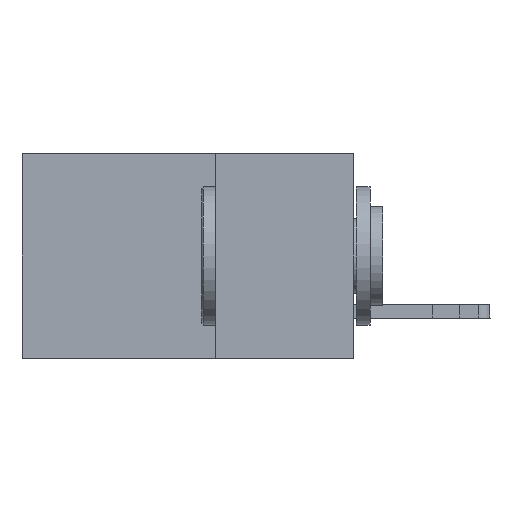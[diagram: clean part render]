
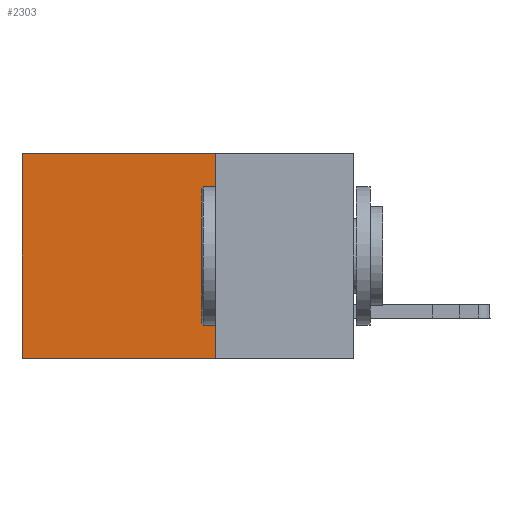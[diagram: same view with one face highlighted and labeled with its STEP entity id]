
A CAD part, left-side view. The second image highlights one B-rep face of the part: STEP entity #2303.
In plain terms, the highlighted planar face has unit normal (-1, 0, 0).
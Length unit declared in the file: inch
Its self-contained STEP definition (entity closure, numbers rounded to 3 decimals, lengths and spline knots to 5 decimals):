
#445 = PLANE ( 'NONE',  #12260 ) ;
#1145 = CARTESIAN_POINT ( 'NONE',  ( 0.2875, 0.25, 0. ) ) ;
#2303 = ADVANCED_FACE ( 'NONE', ( #20921 ), #445, .F. ) ;
#3316 = CARTESIAN_POINT ( 'NONE',  ( 0.2875, 0.25, 0. ) ) ;
#3479 = CARTESIAN_POINT ( 'NONE',  ( 0.2875, 0.6, 0. ) ) ;
#4446 = LINE ( 'NONE', #1145, #18919 ) ;
#5139 = VECTOR ( 'NONE', #6202, 39.37008 ) ;
#5223 = CARTESIAN_POINT ( 'NONE',  ( 0.2875, 0.25, 0. ) ) ;
#6024 = DIRECTION ( 'NONE',  ( 1., 0., 0. ) ) ;
#6202 = DIRECTION ( 'NONE',  ( 0., 0., -1. ) ) ;
#6654 = EDGE_CURVE ( 'NONE', #11622, #7155, #20971, .T. ) ;
#7155 = VERTEX_POINT ( 'NONE', #7326 ) ;
#7326 = CARTESIAN_POINT ( 'NONE',  ( 0.2875, 0.6, 0. ) ) ;
#7704 = ORIENTED_EDGE ( 'NONE', *, *, #6654, .T. ) ;
#9052 = LINE ( 'NONE', #23114, #22618 ) ;
#11622 = VERTEX_POINT ( 'NONE', #21264 ) ;
#12260 = AXIS2_PLACEMENT_3D ( 'NONE', #3316, #6024, #25015 ) ;
#12899 = EDGE_CURVE ( 'NONE', #11622, #27328, #4446, .T. ) ;
#13252 = ORIENTED_EDGE ( 'NONE', *, *, #26945, .T. ) ;
#18919 = VECTOR ( 'NONE', #20245, 39.37008 ) ;
#18921 = DIRECTION ( 'NONE',  ( 0., 1., 0. ) ) ;
#20245 = DIRECTION ( 'NONE',  ( 0., 0., -1. ) ) ;
#20431 = ORIENTED_EDGE ( 'NONE', *, *, #25728, .F. ) ;
#20921 = FACE_OUTER_BOUND ( 'NONE', #31967, .T. ) ;
#20971 = LINE ( 'NONE', #5223, #27322 ) ;
#21264 = CARTESIAN_POINT ( 'NONE',  ( 0.2875, 0.25, 0. ) ) ;
#21280 = ORIENTED_EDGE ( 'NONE', *, *, #12899, .F. ) ;
#22618 = VECTOR ( 'NONE', #25848, 39.37008 ) ;
#23114 = CARTESIAN_POINT ( 'NONE',  ( 0.2875, 0.25, -0.37 ) ) ;
#25015 = DIRECTION ( 'NONE',  ( 0., 0., -1. ) ) ;
#25728 = EDGE_CURVE ( 'NONE', #27328, #35174, #9052, .T. ) ;
#25848 = DIRECTION ( 'NONE',  ( 0., 1., 0. ) ) ;
#26788 = LINE ( 'NONE', #3479, #5139 ) ;
#26945 = EDGE_CURVE ( 'NONE', #7155, #35174, #26788, .T. ) ;
#27322 = VECTOR ( 'NONE', #18921, 39.37008 ) ;
#27328 = VERTEX_POINT ( 'NONE', #34721 ) ;
#31166 = CARTESIAN_POINT ( 'NONE',  ( 0.2875, 0.6, -0.37 ) ) ;
#31967 = EDGE_LOOP ( 'NONE', ( #13252, #20431, #21280, #7704 ) ) ;
#34721 = CARTESIAN_POINT ( 'NONE',  ( 0.2875, 0.25, -0.37 ) ) ;
#35174 = VERTEX_POINT ( 'NONE', #31166 ) ;
